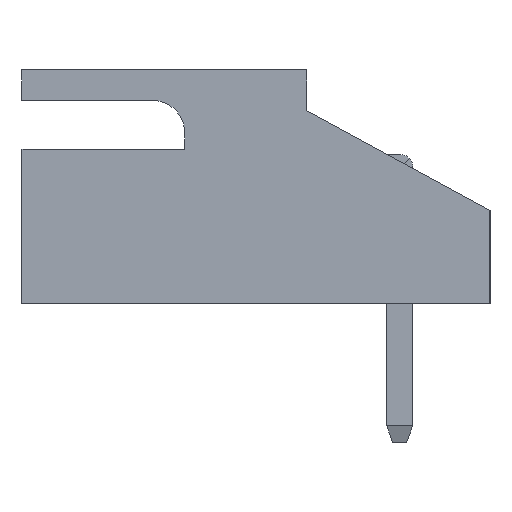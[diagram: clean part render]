
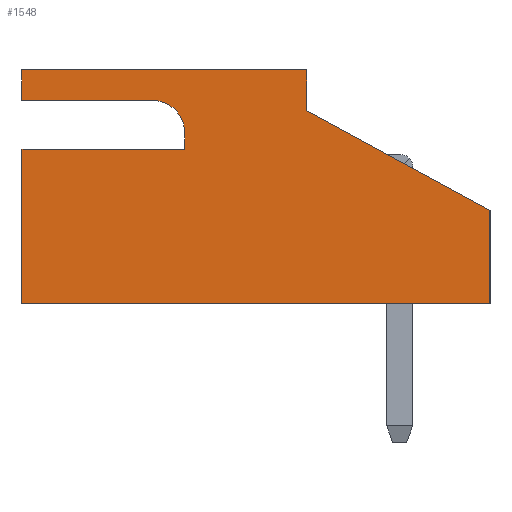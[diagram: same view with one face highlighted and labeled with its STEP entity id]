
A CAD part, left-side view. The second image highlights one B-rep face of the part: STEP entity #1548.
In plain terms, the highlighted planar face has unit normal (-1, 0, 0).
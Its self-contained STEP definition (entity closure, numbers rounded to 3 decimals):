
#65 = DIRECTION ( 'NONE',  ( 0., -1., 0. ) ) ;
#96 = VERTEX_POINT ( 'NONE', #375 ) ;
#135 = VECTOR ( 'NONE', #553, 1000. ) ;
#170 = LINE ( 'NONE', #523, #4774 ) ;
#242 = ORIENTED_EDGE ( 'NONE', *, *, #1292, .T. ) ;
#264 = EDGE_CURVE ( 'NONE', #4803, #4902, #170, .T. ) ;
#352 = CARTESIAN_POINT ( 'NONE',  ( -10., 7., 2.125 ) ) ;
#372 = VECTOR ( 'NONE', #4626, 1000. ) ;
#375 = CARTESIAN_POINT ( 'NONE',  ( -10., 7., 2.875 ) ) ;
#439 = CARTESIAN_POINT ( 'NONE',  ( -10., 7., 2.875 ) ) ;
#477 = EDGE_CURVE ( 'NONE', #820, #920, #1357, .T. ) ;
#502 = EDGE_CURVE ( 'NONE', #920, #1823, #2579, .T. ) ;
#523 = CARTESIAN_POINT ( 'NONE',  ( -10., 7., -2.875 ) ) ;
#533 = VECTOR ( 'NONE', #4521, 1000. ) ;
#553 = DIRECTION ( 'NONE',  ( 0., 0., -1. ) ) ;
#586 = VERTEX_POINT ( 'NONE', #2283 ) ;
#718 = EDGE_CURVE ( 'NONE', #586, #1826, #3581, .T. ) ;
#820 = VERTEX_POINT ( 'NONE', #4847 ) ;
#906 = DIRECTION ( 'NONE',  ( 0., 0., 1. ) ) ;
#920 = VERTEX_POINT ( 'NONE', #1479 ) ;
#995 = VECTOR ( 'NONE', #2086, 1000. ) ;
#1008 = AXIS2_PLACEMENT_3D ( 'NONE', #1726, #1453, #1804 ) ;
#1051 = CARTESIAN_POINT ( 'NONE',  ( -10., 0., -2.875 ) ) ;
#1112 = EDGE_CURVE ( 'NONE', #3561, #586, #2989, .T. ) ;
#1156 = ORIENTED_EDGE ( 'NONE', *, *, #2477, .T. ) ;
#1205 = EDGE_LOOP ( 'NONE', ( #2018, #2410, #4153, #1791, #242, #1277, #1156, #4036, #4410, #2241, #4820 ) ) ;
#1265 = EDGE_CURVE ( 'NONE', #3561, #96, #2888, .T. ) ;
#1277 = ORIENTED_EDGE ( 'NONE', *, *, #264, .F. ) ;
#1292 = EDGE_CURVE ( 'NONE', #4601, #4902, #3401, .T. ) ;
#1298 = CARTESIAN_POINT ( 'NONE',  ( -10., 3., 0.925 ) ) ;
#1357 = LINE ( 'NONE', #3999, #995 ) ;
#1411 = CARTESIAN_POINT ( 'NONE',  ( -10., 3., 1.325 ) ) ;
#1453 = DIRECTION ( 'NONE',  ( 1., 0., 0. ) ) ;
#1479 = CARTESIAN_POINT ( 'NONE',  ( -10., -4.5, -0.575 ) ) ;
#1548 = ADVANCED_FACE ( 'NONE', ( #3351 ), #2670, .F. ) ;
#1726 = CARTESIAN_POINT ( 'NONE',  ( -10., 3.8, 1.325 ) ) ;
#1785 = LINE ( 'NONE', #3979, #135 ) ;
#1791 = ORIENTED_EDGE ( 'NONE', *, *, #1861, .T. ) ;
#1795 = VECTOR ( 'NONE', #2524, 1000. ) ;
#1804 = DIRECTION ( 'NONE',  ( 0., 0., -1. ) ) ;
#1823 = VERTEX_POINT ( 'NONE', #2067 ) ;
#1826 = VERTEX_POINT ( 'NONE', #1411 ) ;
#1861 = EDGE_CURVE ( 'NONE', #1826, #4601, #1785, .T. ) ;
#1901 = CARTESIAN_POINT ( 'NONE',  ( -10., 7., -2.875 ) ) ;
#2018 = ORIENTED_EDGE ( 'NONE', *, *, #1265, .F. ) ;
#2067 = CARTESIAN_POINT ( 'NONE',  ( -10., -4.5, -2.875 ) ) ;
#2086 = DIRECTION ( 'NONE',  ( 0., -0.878, -0.478 ) ) ;
#2241 = ORIENTED_EDGE ( 'NONE', *, *, #2822, .T. ) ;
#2245 = VECTOR ( 'NONE', #3046, 1000. ) ;
#2283 = CARTESIAN_POINT ( 'NONE',  ( -10., 3.8, 2.125 ) ) ;
#2321 = DIRECTION ( 'NONE',  ( 0., 0., -1. ) ) ;
#2401 = CARTESIAN_POINT ( 'NONE',  ( -10., 7., -2.875 ) ) ;
#2410 = ORIENTED_EDGE ( 'NONE', *, *, #1112, .T. ) ;
#2477 = EDGE_CURVE ( 'NONE', #4803, #1823, #3850, .T. ) ;
#2524 = DIRECTION ( 'NONE',  ( 0., 0., 1. ) ) ;
#2528 = AXIS2_PLACEMENT_3D ( 'NONE', #4887, #2699, #2321 ) ;
#2537 = DIRECTION ( 'NONE',  ( 0., 0., 1. ) ) ;
#2546 = LINE ( 'NONE', #1051, #1795 ) ;
#2579 = LINE ( 'NONE', #2981, #533 ) ;
#2670 = PLANE ( 'NONE',  #2528 ) ;
#2699 = DIRECTION ( 'NONE',  ( 1., 0., 0. ) ) ;
#2822 = EDGE_CURVE ( 'NONE', #820, #4645, #2546, .T. ) ;
#2888 = LINE ( 'NONE', #4432, #3290 ) ;
#2974 = EDGE_CURVE ( 'NONE', #96, #4645, #3055, .T. ) ;
#2981 = CARTESIAN_POINT ( 'NONE',  ( -10., -4.5, -0.575 ) ) ;
#2989 = LINE ( 'NONE', #352, #4340 ) ;
#2995 = CARTESIAN_POINT ( 'NONE',  ( -10., 0., 2.875 ) ) ;
#3046 = DIRECTION ( 'NONE',  ( 0., 1., 0. ) ) ;
#3055 = LINE ( 'NONE', #439, #3966 ) ;
#3290 = VECTOR ( 'NONE', #2537, 1000. ) ;
#3351 = FACE_OUTER_BOUND ( 'NONE', #1205, .T. ) ;
#3401 = LINE ( 'NONE', #4941, #2245 ) ;
#3561 = VERTEX_POINT ( 'NONE', #3648 ) ;
#3581 = CIRCLE ( 'NONE', #1008, 0.8 ) ;
#3648 = CARTESIAN_POINT ( 'NONE',  ( -10., 7., 2.125 ) ) ;
#3850 = LINE ( 'NONE', #2401, #372 ) ;
#3966 = VECTOR ( 'NONE', #65, 1000. ) ;
#3979 = CARTESIAN_POINT ( 'NONE',  ( -10., 3., 1.325 ) ) ;
#3999 = CARTESIAN_POINT ( 'NONE',  ( -10., 0., 1.875 ) ) ;
#4036 = ORIENTED_EDGE ( 'NONE', *, *, #502, .F. ) ;
#4153 = ORIENTED_EDGE ( 'NONE', *, *, #718, .T. ) ;
#4340 = VECTOR ( 'NONE', #4529, 1000. ) ;
#4410 = ORIENTED_EDGE ( 'NONE', *, *, #477, .F. ) ;
#4432 = CARTESIAN_POINT ( 'NONE',  ( -10., 7., -2.875 ) ) ;
#4521 = DIRECTION ( 'NONE',  ( 0., 0., -1. ) ) ;
#4529 = DIRECTION ( 'NONE',  ( 0., -1., 0. ) ) ;
#4601 = VERTEX_POINT ( 'NONE', #1298 ) ;
#4615 = CARTESIAN_POINT ( 'NONE',  ( -10., 7., 0.925 ) ) ;
#4626 = DIRECTION ( 'NONE',  ( 0., -1., 0. ) ) ;
#4645 = VERTEX_POINT ( 'NONE', #2995 ) ;
#4774 = VECTOR ( 'NONE', #906, 1000. ) ;
#4803 = VERTEX_POINT ( 'NONE', #1901 ) ;
#4820 = ORIENTED_EDGE ( 'NONE', *, *, #2974, .F. ) ;
#4847 = CARTESIAN_POINT ( 'NONE',  ( -10., 0., 1.875 ) ) ;
#4887 = CARTESIAN_POINT ( 'NONE',  ( -10., 7., -2.875 ) ) ;
#4902 = VERTEX_POINT ( 'NONE', #4615 ) ;
#4941 = CARTESIAN_POINT ( 'NONE',  ( -10., 7., 0.925 ) ) ;
